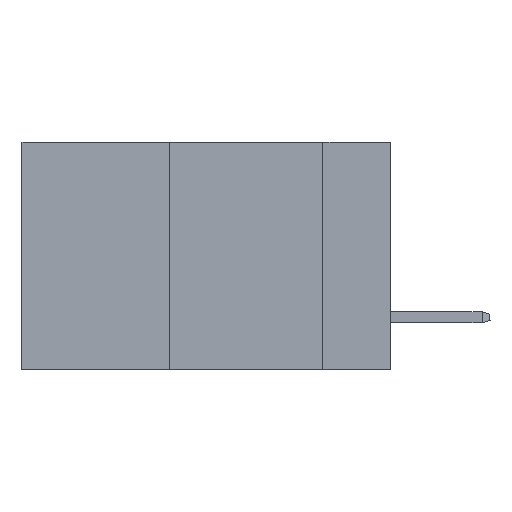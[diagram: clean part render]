
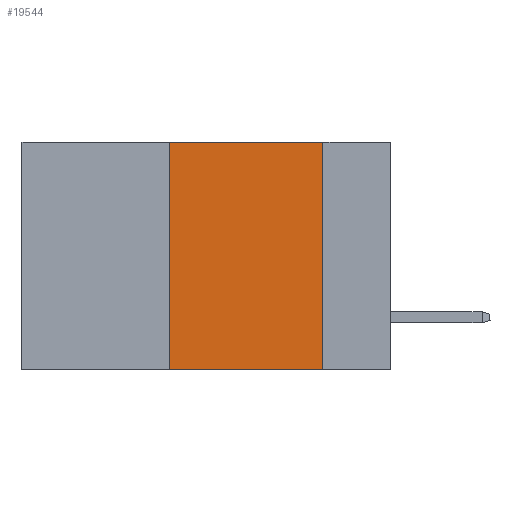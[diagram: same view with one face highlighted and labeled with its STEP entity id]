
A CAD part, left-side view. The second image highlights one B-rep face of the part: STEP entity #19544.
In plain terms, the highlighted planar face has unit normal (-1, 0, 0).
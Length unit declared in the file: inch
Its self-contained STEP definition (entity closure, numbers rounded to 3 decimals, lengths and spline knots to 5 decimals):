
#589 = FACE_OUTER_BOUND ( 'NONE', #10430, .T. ) ;
#789 = EDGE_CURVE ( 'NONE', #11424, #24386, #20746, .T. ) ;
#4059 = EDGE_CURVE ( 'NONE', #35056, #11424, #35178, .T. ) ;
#6115 = CARTESIAN_POINT ( 'NONE',  ( 0., 0.6, -0.37 ) ) ;
#9823 = DIRECTION ( 'NONE',  ( 1., 0., 0. ) ) ;
#9955 = CARTESIAN_POINT ( 'NONE',  ( 0., 0.6, 0. ) ) ;
#10430 = EDGE_LOOP ( 'NONE', ( #25854, #30507, #19894, #11017 ) ) ;
#11017 = ORIENTED_EDGE ( 'NONE', *, *, #11920, .T. ) ;
#11424 = VERTEX_POINT ( 'NONE', #11999 ) ;
#11920 = EDGE_CURVE ( 'NONE', #35056, #18060, #25685, .T. ) ;
#11999 = CARTESIAN_POINT ( 'NONE',  ( 0., 0.36, 0. ) ) ;
#13689 = VECTOR ( 'NONE', #20496, 39.37008 ) ;
#16790 = EDGE_CURVE ( 'NONE', #24386, #18060, #20965, .T. ) ;
#17734 = CARTESIAN_POINT ( 'NONE',  ( 0., 0.6, 0. ) ) ;
#18060 = VERTEX_POINT ( 'NONE', #31451 ) ;
#19241 = AXIS2_PLACEMENT_3D ( 'NONE', #9955, #9823, #39688 ) ;
#19544 = ADVANCED_FACE ( 'NONE', ( #589 ), #26473, .F. ) ;
#19894 = ORIENTED_EDGE ( 'NONE', *, *, #4059, .F. ) ;
#20496 = DIRECTION ( 'NONE',  ( 0., -1., 0. ) ) ;
#20746 = LINE ( 'NONE', #17734, #29597 ) ;
#20965 = LINE ( 'NONE', #33533, #27165 ) ;
#21946 = DIRECTION ( 'NONE',  ( 0., 0., 1. ) ) ;
#23856 = DIRECTION ( 'NONE',  ( 0., -1., 0. ) ) ;
#24386 = VERTEX_POINT ( 'NONE', #28353 ) ;
#25410 = CARTESIAN_POINT ( 'NONE',  ( 0., 0.36, 0. ) ) ;
#25685 = LINE ( 'NONE', #6115, #13689 ) ;
#25854 = ORIENTED_EDGE ( 'NONE', *, *, #16790, .F. ) ;
#26473 = PLANE ( 'NONE',  #19241 ) ;
#27165 = VECTOR ( 'NONE', #28723, 39.37008 ) ;
#28051 = CARTESIAN_POINT ( 'NONE',  ( 0., 0.36, -0.37 ) ) ;
#28353 = CARTESIAN_POINT ( 'NONE',  ( 0., 0.11, 0. ) ) ;
#28723 = DIRECTION ( 'NONE',  ( 0., 0., -1. ) ) ;
#29597 = VECTOR ( 'NONE', #23856, 39.37008 ) ;
#30507 = ORIENTED_EDGE ( 'NONE', *, *, #789, .F. ) ;
#30542 = VECTOR ( 'NONE', #21946, 39.37008 ) ;
#31451 = CARTESIAN_POINT ( 'NONE',  ( 0., 0.11, -0.37 ) ) ;
#33533 = CARTESIAN_POINT ( 'NONE',  ( 0., 0.11, 0. ) ) ;
#35056 = VERTEX_POINT ( 'NONE', #28051 ) ;
#35178 = LINE ( 'NONE', #25410, #30542 ) ;
#39688 = DIRECTION ( 'NONE',  ( 0., 0., -1. ) ) ;
